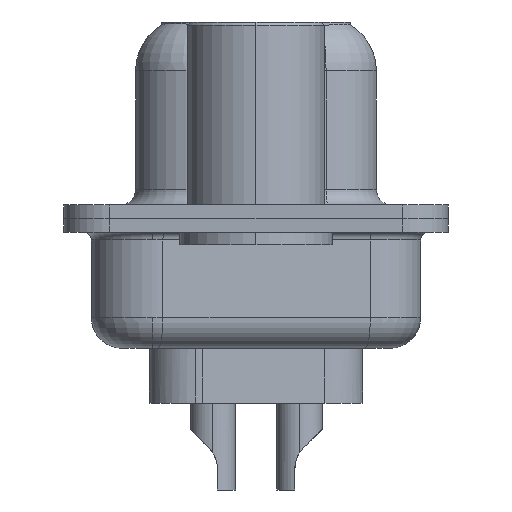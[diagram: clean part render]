
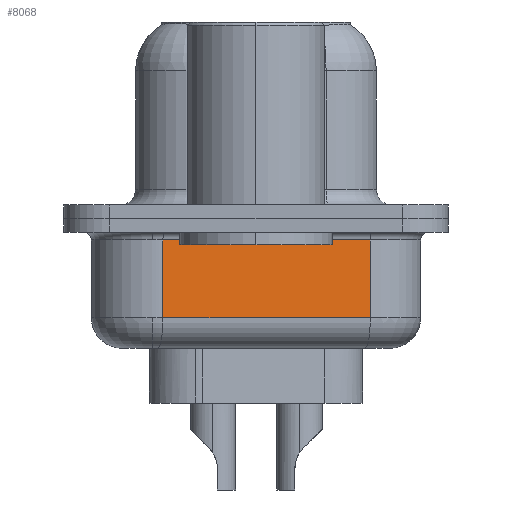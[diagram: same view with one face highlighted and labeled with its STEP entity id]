
A CAD part, left-side view. The second image highlights one B-rep face of the part: STEP entity #8068.
In plain terms, the highlighted planar face has unit normal (-0.985, -0.174, 0).
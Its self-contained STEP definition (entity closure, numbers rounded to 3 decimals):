
#435 = VERTEX_POINT ( 'NONE', #4514 ) ;
#564 = ORIENTED_EDGE ( 'NONE', *, *, #18278, .T. ) ;
#962 = CARTESIAN_POINT ( 'NONE',  ( 4.049, -3.747, -4.25 ) ) ;
#993 = CARTESIAN_POINT ( 'NONE',  ( 2.85, 3.053, -3.25 ) ) ;
#998 = EDGE_CURVE ( 'NONE', #435, #25939, #25221, .T. ) ;
#1538 = DIRECTION ( 'NONE',  ( -0.174, 0.985, 0. ) ) ;
#1547 = CARTESIAN_POINT ( 'NONE',  ( 4.049, -3.747, -0.7 ) ) ;
#2975 = ORIENTED_EDGE ( 'NONE', *, *, #998, .T. ) ;
#3541 = CARTESIAN_POINT ( 'NONE',  ( 2.85, 3.053, -4.25 ) ) ;
#3840 = AXIS2_PLACEMENT_3D ( 'NONE', #3541, #25899, #1538 ) ;
#4027 = EDGE_CURVE ( 'NONE', #9531, #13908, #12045, .T. ) ;
#4514 = CARTESIAN_POINT ( 'NONE',  ( 2.85, 3.053, -3.25 ) ) ;
#7397 = DIRECTION ( 'NONE',  ( 0.174, -0.985, 0. ) ) ;
#8068 = ADVANCED_FACE ( 'NONE', ( #9938 ), #26039, .F. ) ;
#8342 = CARTESIAN_POINT ( 'NONE',  ( 2.85, 3.053, -4.25 ) ) ;
#9531 = VERTEX_POINT ( 'NONE', #1547 ) ;
#9938 = FACE_OUTER_BOUND ( 'NONE', #10101, .T. ) ;
#10101 = EDGE_LOOP ( 'NONE', ( #18603, #2975, #564, #25186 ) ) ;
#10894 = CARTESIAN_POINT ( 'NONE',  ( 4.049, -3.747, -3.25 ) ) ;
#12045 = LINE ( 'NONE', #14026, #20280 ) ;
#13908 = VERTEX_POINT ( 'NONE', #25541 ) ;
#14026 = CARTESIAN_POINT ( 'NONE',  ( 2.85, 3.053, -0.7 ) ) ;
#14378 = VECTOR ( 'NONE', #21571, 1000. ) ;
#17601 = DIRECTION ( 'NONE',  ( -0.174, 0.985, 0. ) ) ;
#18278 = EDGE_CURVE ( 'NONE', #25939, #9531, #21036, .T. ) ;
#18492 = VECTOR ( 'NONE', #7397, 1000. ) ;
#18603 = ORIENTED_EDGE ( 'NONE', *, *, #22347, .F. ) ;
#20280 = VECTOR ( 'NONE', #17601, 1000. ) ;
#21036 = LINE ( 'NONE', #962, #14378 ) ;
#21571 = DIRECTION ( 'NONE',  ( 0., 0., 1. ) ) ;
#22347 = EDGE_CURVE ( 'NONE', #435, #13908, #25457, .T. ) ;
#22573 = DIRECTION ( 'NONE',  ( 0., 0., 1. ) ) ;
#24675 = VECTOR ( 'NONE', #22573, 1000. ) ;
#25186 = ORIENTED_EDGE ( 'NONE', *, *, #4027, .T. ) ;
#25221 = LINE ( 'NONE', #993, #18492 ) ;
#25457 = LINE ( 'NONE', #8342, #24675 ) ;
#25541 = CARTESIAN_POINT ( 'NONE',  ( 2.85, 3.053, -0.7 ) ) ;
#25899 = DIRECTION ( 'NONE',  ( 0.985, 0.174, 0. ) ) ;
#25939 = VERTEX_POINT ( 'NONE', #10894 ) ;
#26039 = PLANE ( 'NONE',  #3840 ) ;
